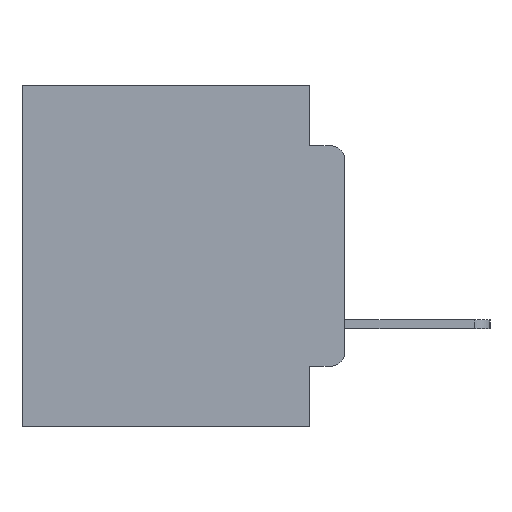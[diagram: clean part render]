
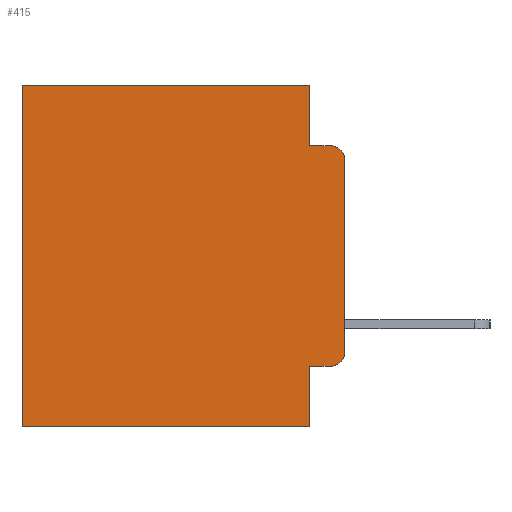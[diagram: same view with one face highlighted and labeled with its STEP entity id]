
A CAD part, left-side view. The second image highlights one B-rep face of the part: STEP entity #415.
In plain terms, the highlighted planar face has unit normal (-1, 0, 0).
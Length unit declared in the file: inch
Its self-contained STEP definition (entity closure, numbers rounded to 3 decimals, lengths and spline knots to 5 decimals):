
#191 = AXIS2_PLACEMENT_3D ( 'NONE', #2310, #17193, #4504 ) ;
#415 = ADVANCED_FACE ( 'NONE', ( #11389 ), #4114, .F. ) ;
#520 = ORIENTED_EDGE ( 'NONE', *, *, #2929, .F. ) ;
#1454 = EDGE_CURVE ( 'NONE', #24588, #25455, #22432, .T. ) ;
#1823 = VERTEX_POINT ( 'NONE', #19828 ) ;
#2310 = CARTESIAN_POINT ( 'NONE',  ( 0.298, 0.02, -0.3915 ) ) ;
#2598 = CARTESIAN_POINT ( 'NONE',  ( 0.298, 0.473, -0.5 ) ) ;
#2929 = EDGE_CURVE ( 'NONE', #1823, #18511, #3087, .T. ) ;
#3087 = LINE ( 'NONE', #4541, #19974 ) ;
#4086 = CIRCLE ( 'NONE', #191, 0.02 ) ;
#4114 = PLANE ( 'NONE',  #20107 ) ;
#4395 = EDGE_CURVE ( 'NONE', #18511, #19420, #12421, .T. ) ;
#4504 = DIRECTION ( 'NONE',  ( 0., 0., -1. ) ) ;
#4541 = CARTESIAN_POINT ( 'NONE',  ( 0.298, 0.051, 0. ) ) ;
#4852 = LINE ( 'NONE', #22465, #26474 ) ;
#5168 = DIRECTION ( 'NONE',  ( 0., 0., -1. ) ) ;
#5194 = CARTESIAN_POINT ( 'NONE',  ( 0.298, 0., 0. ) ) ;
#5255 = VERTEX_POINT ( 'NONE', #23401 ) ;
#5799 = CARTESIAN_POINT ( 'NONE',  ( 0.298, 0.051, -0.4115 ) ) ;
#5896 = EDGE_CURVE ( 'NONE', #9540, #19420, #9697, .T. ) ;
#6247 = DIRECTION ( 'NONE',  ( 1., 0., 0. ) ) ;
#6498 = AXIS2_PLACEMENT_3D ( 'NONE', #9156, #23730, #11252 ) ;
#6795 = VECTOR ( 'NONE', #19702, 39.37008 ) ;
#7246 = CARTESIAN_POINT ( 'NONE',  ( 0.298, 0.473, 0. ) ) ;
#7547 = CARTESIAN_POINT ( 'NONE',  ( 0.298, 0.051, 0. ) ) ;
#7744 = VERTEX_POINT ( 'NONE', #25339 ) ;
#7760 = ORIENTED_EDGE ( 'NONE', *, *, #1454, .T. ) ;
#8780 = EDGE_CURVE ( 'NONE', #9540, #5255, #4852, .T. ) ;
#9104 = ORIENTED_EDGE ( 'NONE', *, *, #27381, .F. ) ;
#9156 = CARTESIAN_POINT ( 'NONE',  ( 0.298, 0.02, -0.1085 ) ) ;
#9180 = CARTESIAN_POINT ( 'NONE',  ( 0.298, 0.051, -0.5 ) ) ;
#9418 = ORIENTED_EDGE ( 'NONE', *, *, #8780, .F. ) ;
#9469 = LINE ( 'NONE', #20724, #20576 ) ;
#9540 = VERTEX_POINT ( 'NONE', #10748 ) ;
#9645 = EDGE_CURVE ( 'NONE', #24130, #25455, #11169, .T. ) ;
#9697 = CIRCLE ( 'NONE', #6498, 0.02 ) ;
#10081 = ORIENTED_EDGE ( 'NONE', *, *, #5896, .T. ) ;
#10662 = VECTOR ( 'NONE', #26315, 39.37008 ) ;
#10748 = CARTESIAN_POINT ( 'NONE',  ( 0.298, 0., -0.1085 ) ) ;
#11169 = LINE ( 'NONE', #13205, #27083 ) ;
#11252 = DIRECTION ( 'NONE',  ( 0., 0., -1. ) ) ;
#11302 = CARTESIAN_POINT ( 'NONE',  ( 0.298, 0.051, -0.0885 ) ) ;
#11389 = FACE_OUTER_BOUND ( 'NONE', #14524, .T. ) ;
#12073 = DIRECTION ( 'NONE',  ( 0., 0., -1. ) ) ;
#12421 = LINE ( 'NONE', #11302, #6795 ) ;
#13205 = CARTESIAN_POINT ( 'NONE',  ( 0.298, 0., -0.5 ) ) ;
#13354 = CARTESIAN_POINT ( 'NONE',  ( 0.298, 0.051, -0.4115 ) ) ;
#14524 = EDGE_LOOP ( 'NONE', ( #9418, #10081, #16945, #520, #23760, #7760, #18912, #9104, #14678, #21531 ) ) ;
#14678 = ORIENTED_EDGE ( 'NONE', *, *, #25995, .T. ) ;
#14927 = CARTESIAN_POINT ( 'NONE',  ( 0.298, 0.473, 0. ) ) ;
#15321 = DIRECTION ( 'NONE',  ( 0., 1., 0. ) ) ;
#15452 = DIRECTION ( 'NONE',  ( 0., -1., 0. ) ) ;
#16038 = VECTOR ( 'NONE', #15452, 39.37008 ) ;
#16887 = VECTOR ( 'NONE', #18882, 39.37008 ) ;
#16945 = ORIENTED_EDGE ( 'NONE', *, *, #4395, .F. ) ;
#17193 = DIRECTION ( 'NONE',  ( -1., 0., 0. ) ) ;
#18511 = VERTEX_POINT ( 'NONE', #19222 ) ;
#18882 = DIRECTION ( 'NONE',  ( 0., 0., -1. ) ) ;
#18912 = ORIENTED_EDGE ( 'NONE', *, *, #9645, .F. ) ;
#19222 = CARTESIAN_POINT ( 'NONE',  ( 0.298, 0.051, -0.0885 ) ) ;
#19420 = VERTEX_POINT ( 'NONE', #20633 ) ;
#19702 = DIRECTION ( 'NONE',  ( 0., -1., 0. ) ) ;
#19828 = CARTESIAN_POINT ( 'NONE',  ( 0.298, 0.051, 0. ) ) ;
#19974 = VECTOR ( 'NONE', #21426, 39.37008 ) ;
#20107 = AXIS2_PLACEMENT_3D ( 'NONE', #5194, #6247, #5168 ) ;
#20576 = VECTOR ( 'NONE', #22835, 39.37008 ) ;
#20633 = CARTESIAN_POINT ( 'NONE',  ( 0.298, 0.02, -0.0885 ) ) ;
#20724 = CARTESIAN_POINT ( 'NONE',  ( 0.298, 0., 0. ) ) ;
#21426 = DIRECTION ( 'NONE',  ( 0., 0., -1. ) ) ;
#21531 = ORIENTED_EDGE ( 'NONE', *, *, #24634, .T. ) ;
#22432 = LINE ( 'NONE', #7246, #16887 ) ;
#22465 = CARTESIAN_POINT ( 'NONE',  ( 0.298, 0., 0. ) ) ;
#22835 = DIRECTION ( 'NONE',  ( 0., 1., 0. ) ) ;
#23401 = CARTESIAN_POINT ( 'NONE',  ( 0.298, 0., -0.3915 ) ) ;
#23730 = DIRECTION ( 'NONE',  ( -1., 0., 0. ) ) ;
#23760 = ORIENTED_EDGE ( 'NONE', *, *, #25827, .T. ) ;
#24130 = VERTEX_POINT ( 'NONE', #9180 ) ;
#24429 = VERTEX_POINT ( 'NONE', #5799 ) ;
#24588 = VERTEX_POINT ( 'NONE', #14927 ) ;
#24634 = EDGE_CURVE ( 'NONE', #7744, #5255, #4086, .T. ) ;
#25339 = CARTESIAN_POINT ( 'NONE',  ( 0.298, 0.02, -0.4115 ) ) ;
#25455 = VERTEX_POINT ( 'NONE', #2598 ) ;
#25827 = EDGE_CURVE ( 'NONE', #1823, #24588, #9469, .T. ) ;
#25995 = EDGE_CURVE ( 'NONE', #24429, #7744, #27006, .T. ) ;
#26315 = DIRECTION ( 'NONE',  ( 0., 0., -1. ) ) ;
#26474 = VECTOR ( 'NONE', #12073, 39.37008 ) ;
#27006 = LINE ( 'NONE', #13354, #16038 ) ;
#27083 = VECTOR ( 'NONE', #15321, 39.37008 ) ;
#27212 = LINE ( 'NONE', #7547, #10662 ) ;
#27381 = EDGE_CURVE ( 'NONE', #24429, #24130, #27212, .T. ) ;
